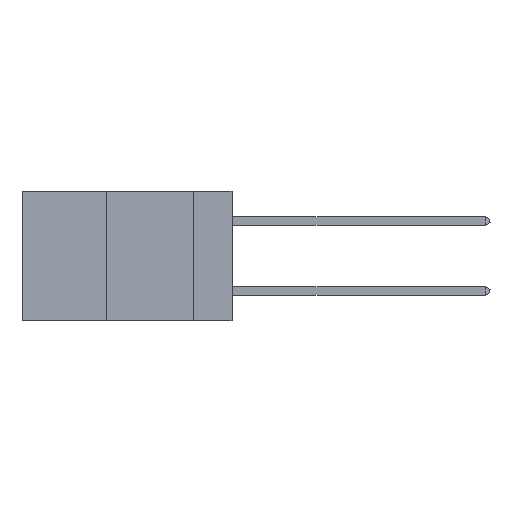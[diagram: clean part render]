
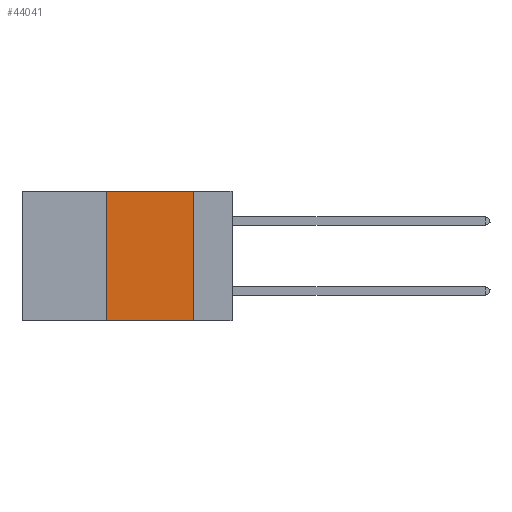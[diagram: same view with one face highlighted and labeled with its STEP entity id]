
A CAD part, left-side view. The second image highlights one B-rep face of the part: STEP entity #44041.
In plain terms, the highlighted planar face has unit normal (-1, 0, 0).
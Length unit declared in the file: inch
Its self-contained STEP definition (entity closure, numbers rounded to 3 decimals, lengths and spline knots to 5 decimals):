
#453 = LINE ( 'NONE', #37019, #42194 ) ;
#1355 = EDGE_CURVE ( 'NONE', #3665, #35894, #453, .T. ) ;
#1609 = AXIS2_PLACEMENT_3D ( 'NONE', #21206, #31956, #10909 ) ;
#2786 = ORIENTED_EDGE ( 'NONE', *, *, #16822, .F. ) ;
#3665 = VERTEX_POINT ( 'NONE', #44849 ) ;
#4526 = CARTESIAN_POINT ( 'NONE',  ( 0., 0.36, 0. ) ) ;
#6442 = ORIENTED_EDGE ( 'NONE', *, *, #31752, .T. ) ;
#6933 = EDGE_LOOP ( 'NONE', ( #37751, #2786, #10555, #6442 ) ) ;
#7512 = VECTOR ( 'NONE', #9610, 39.37008 ) ;
#8153 = CARTESIAN_POINT ( 'NONE',  ( 0., 0.36, -0.37 ) ) ;
#8469 = LINE ( 'NONE', #16630, #44123 ) ;
#9610 = DIRECTION ( 'NONE',  ( 0., -1., 0. ) ) ;
#9720 = DIRECTION ( 'NONE',  ( 0., 0., 1. ) ) ;
#10555 = ORIENTED_EDGE ( 'NONE', *, *, #10688, .F. ) ;
#10688 = EDGE_CURVE ( 'NONE', #43409, #11671, #8469, .T. ) ;
#10909 = DIRECTION ( 'NONE',  ( 0., 0., -1. ) ) ;
#11048 = PLANE ( 'NONE',  #1609 ) ;
#11671 = VERTEX_POINT ( 'NONE', #4526 ) ;
#11933 = DIRECTION ( 'NONE',  ( 0., -1., 0. ) ) ;
#12541 = CARTESIAN_POINT ( 'NONE',  ( 0., 0.11, -0.37 ) ) ;
#16630 = CARTESIAN_POINT ( 'NONE',  ( 0., 0.36, 0. ) ) ;
#16822 = EDGE_CURVE ( 'NONE', #11671, #3665, #40455, .T. ) ;
#18500 = LINE ( 'NONE', #29904, #22316 ) ;
#21206 = CARTESIAN_POINT ( 'NONE',  ( 0., 0.6, 0. ) ) ;
#22316 = VECTOR ( 'NONE', #11933, 39.37008 ) ;
#27105 = CARTESIAN_POINT ( 'NONE',  ( 0., 0.6, 0. ) ) ;
#29904 = CARTESIAN_POINT ( 'NONE',  ( 0., 0.6, -0.37 ) ) ;
#31752 = EDGE_CURVE ( 'NONE', #43409, #35894, #18500, .T. ) ;
#31956 = DIRECTION ( 'NONE',  ( 1., 0., 0. ) ) ;
#32132 = FACE_OUTER_BOUND ( 'NONE', #6933, .T. ) ;
#35894 = VERTEX_POINT ( 'NONE', #12541 ) ;
#37019 = CARTESIAN_POINT ( 'NONE',  ( 0., 0.11, 0. ) ) ;
#37751 = ORIENTED_EDGE ( 'NONE', *, *, #1355, .F. ) ;
#40455 = LINE ( 'NONE', #27105, #7512 ) ;
#42194 = VECTOR ( 'NONE', #43904, 39.37008 ) ;
#43409 = VERTEX_POINT ( 'NONE', #8153 ) ;
#43904 = DIRECTION ( 'NONE',  ( 0., 0., -1. ) ) ;
#44041 = ADVANCED_FACE ( 'NONE', ( #32132 ), #11048, .F. ) ;
#44123 = VECTOR ( 'NONE', #9720, 39.37008 ) ;
#44849 = CARTESIAN_POINT ( 'NONE',  ( 0., 0.11, 0. ) ) ;
